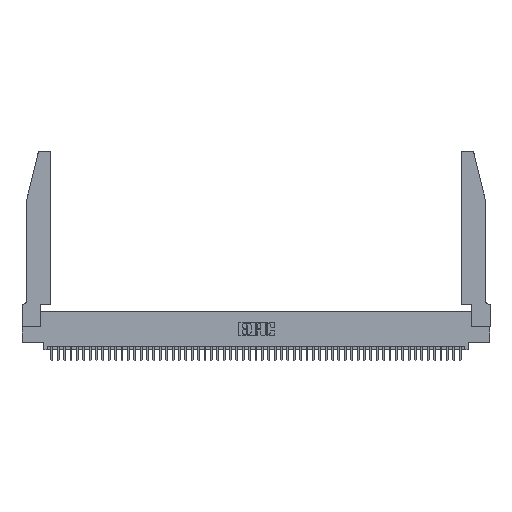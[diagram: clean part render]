
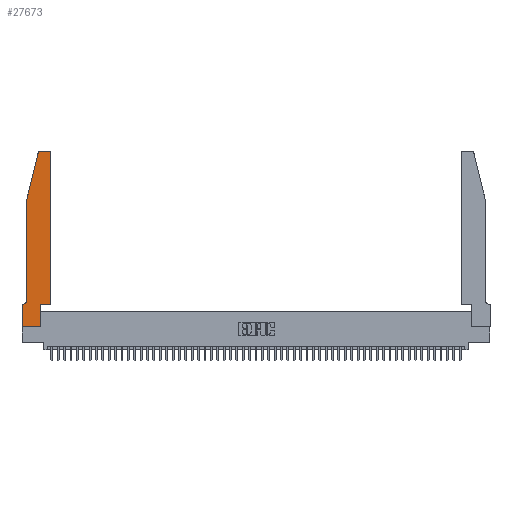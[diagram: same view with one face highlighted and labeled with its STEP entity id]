
A CAD part, top view. The second image highlights one B-rep face of the part: STEP entity #27673.
In plain terms, the highlighted planar face has unit normal (0, 0, 1).
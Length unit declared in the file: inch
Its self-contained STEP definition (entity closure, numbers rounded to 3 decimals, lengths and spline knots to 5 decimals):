
#548 = EDGE_CURVE ( 'NONE', #37580, #27733, #16621, .T. ) ;
#1304 = EDGE_CURVE ( 'NONE', #19321, #5507, #36340, .T. ) ;
#1772 = AXIS2_PLACEMENT_3D ( 'NONE', #45764, #21331, #49885 ) ;
#3377 = EDGE_CURVE ( 'NONE', #11514, #19321, #48997, .T. ) ;
#3870 = EDGE_CURVE ( 'NONE', #5507, #52704, #7978, .T. ) ;
#3989 = ORIENTED_EDGE ( 'NONE', *, *, #1304, .T. ) ;
#4039 = PLANE ( 'NONE',  #30158 ) ;
#5288 = EDGE_CURVE ( 'NONE', #27767, #37580, #44974, .T. ) ;
#5365 = EDGE_CURVE ( 'NONE', #30764, #27767, #31536, .T. ) ;
#5507 = VERTEX_POINT ( 'NONE', #20300 ) ;
#6475 = DIRECTION ( 'NONE',  ( 0., -1., 0. ) ) ;
#6552 = CARTESIAN_POINT ( 'NONE',  ( 0.4205, 2.75, 0.37 ) ) ;
#6656 = EDGE_CURVE ( 'NONE', #52704, #35107, #7088, .T. ) ;
#6718 = VERTEX_POINT ( 'NONE', #19467 ) ;
#7007 = CARTESIAN_POINT ( 'NONE',  ( 0., 0., 0.37 ) ) ;
#7088 = LINE ( 'NONE', #47504, #27619 ) ;
#7978 = CIRCLE ( 'NONE', #17635, 0.03 ) ;
#8817 = LINE ( 'NONE', #20969, #19744 ) ;
#9287 = ORIENTED_EDGE ( 'NONE', *, *, #5288, .T. ) ;
#9328 = ORIENTED_EDGE ( 'NONE', *, *, #3870, .T. ) ;
#9460 = CIRCLE ( 'NONE', #1772, 0.07 ) ;
#9462 = DIRECTION ( 'NONE',  ( 0., 0., 1. ) ) ;
#10316 = ORIENTED_EDGE ( 'NONE', *, *, #6656, .T. ) ;
#10530 = EDGE_CURVE ( 'NONE', #27733, #11514, #35978, .T. ) ;
#11138 = DIRECTION ( 'NONE',  ( 1., 0., 0. ) ) ;
#11514 = VERTEX_POINT ( 'NONE', #12403 ) ;
#11922 = CARTESIAN_POINT ( 'NONE',  ( 0.0755, 2., 0.37 ) ) ;
#12154 = ORIENTED_EDGE ( 'NONE', *, *, #10530, .T. ) ;
#12274 = CARTESIAN_POINT ( 'NONE',  ( 0., 0.35, 0.37 ) ) ;
#12403 = CARTESIAN_POINT ( 'NONE',  ( 0.4505, 2.72, 0.37 ) ) ;
#12608 = ORIENTED_EDGE ( 'NONE', *, *, #48501, .T. ) ;
#12703 = DIRECTION ( 'NONE',  ( -1., 0., 0. ) ) ;
#12795 = CARTESIAN_POINT ( 'NONE',  ( 0.4505, 0.35, 0.37 ) ) ;
#13423 = ORIENTED_EDGE ( 'NONE', *, *, #548, .T. ) ;
#13447 = ORIENTED_EDGE ( 'NONE', *, *, #5365, .T. ) ;
#14265 = VECTOR ( 'NONE', #16942, 39.37008 ) ;
#14744 = DIRECTION ( 'NONE',  ( 0., 0., 1. ) ) ;
#15454 = VERTEX_POINT ( 'NONE', #48443 ) ;
#16170 = CARTESIAN_POINT ( 'NONE',  ( 0.0755, 2., 0.37 ) ) ;
#16423 = DIRECTION ( 'NONE',  ( 1., 0., 0. ) ) ;
#16621 = LINE ( 'NONE', #50655, #37054 ) ;
#16942 = DIRECTION ( 'NONE',  ( 0., 1., 0. ) ) ;
#17635 = AXIS2_PLACEMENT_3D ( 'NONE', #33998, #9462, #38089 ) ;
#18958 = CARTESIAN_POINT ( 'NONE',  ( 0., 0., 0.37 ) ) ;
#18977 = EDGE_CURVE ( 'NONE', #6718, #42644, #8817, .T. ) ;
#19074 = DIRECTION ( 'NONE',  ( 0., 1., 0. ) ) ;
#19321 = VERTEX_POINT ( 'NONE', #6552 ) ;
#19467 = CARTESIAN_POINT ( 'NONE',  ( 0.0055, 0.35, 0.37 ) ) ;
#19744 = VECTOR ( 'NONE', #12703, 39.37008 ) ;
#19857 = LINE ( 'NONE', #16170, #39004 ) ;
#20300 = CARTESIAN_POINT ( 'NONE',  ( 0.284, 2.75, 0.37 ) ) ;
#20580 = CARTESIAN_POINT ( 'NONE',  ( 0.25487, 2.72718, 0.37 ) ) ;
#20799 = FACE_OUTER_BOUND ( 'NONE', #48003, .T. ) ;
#20892 = CARTESIAN_POINT ( 'NONE',  ( 0.2865, 0., 0.37 ) ) ;
#20969 = CARTESIAN_POINT ( 'NONE',  ( 0.0755, 0.35, 0.37 ) ) ;
#21331 = DIRECTION ( 'NONE',  ( 0., 0., -1. ) ) ;
#23020 = CARTESIAN_POINT ( 'NONE',  ( 0.2865, 0.35, 0.37 ) ) ;
#23251 = VECTOR ( 'NONE', #19074, 39.37008 ) ;
#24206 = VECTOR ( 'NONE', #26511, 39.37008 ) ;
#24578 = EDGE_CURVE ( 'NONE', #35107, #15454, #19857, .T. ) ;
#26511 = DIRECTION ( 'NONE',  ( -1., 0., 0. ) ) ;
#26944 = CARTESIAN_POINT ( 'NONE',  ( 0., 0., 0.37 ) ) ;
#27619 = VECTOR ( 'NONE', #43426, 39.37008 ) ;
#27673 = ADVANCED_FACE ( 'NONE', ( #20799 ), #4039, .T. ) ;
#27733 = VERTEX_POINT ( 'NONE', #41225 ) ;
#27767 = VERTEX_POINT ( 'NONE', #20892 ) ;
#28101 = EDGE_CURVE ( 'NONE', #42644, #30764, #41975, .T. ) ;
#30158 = AXIS2_PLACEMENT_3D ( 'NONE', #12274, #40871, #16423 ) ;
#30764 = VERTEX_POINT ( 'NONE', #18958 ) ;
#31098 = VECTOR ( 'NONE', #6475, 39.37008 ) ;
#31536 = LINE ( 'NONE', #7007, #51976 ) ;
#33998 = CARTESIAN_POINT ( 'NONE',  ( 0.284, 2.72, 0.37 ) ) ;
#34607 = CARTESIAN_POINT ( 'NONE',  ( 0., 0.35, 0.37 ) ) ;
#34696 = CARTESIAN_POINT ( 'NONE',  ( 0.2605, 2.75, 0.37 ) ) ;
#35107 = VERTEX_POINT ( 'NONE', #11922 ) ;
#35978 = LINE ( 'NONE', #12795, #14265 ) ;
#36061 = AXIS2_PLACEMENT_3D ( 'NONE', #39190, #14744, #43337 ) ;
#36340 = LINE ( 'NONE', #34696, #24206 ) ;
#37054 = VECTOR ( 'NONE', #46540, 39.37008 ) ;
#37580 = VERTEX_POINT ( 'NONE', #47078 ) ;
#38089 = DIRECTION ( 'NONE',  ( 1., 0., 0. ) ) ;
#39004 = VECTOR ( 'NONE', #48824, 39.37008 ) ;
#39190 = CARTESIAN_POINT ( 'NONE',  ( 0.4205, 2.72, 0.37 ) ) ;
#40871 = DIRECTION ( 'NONE',  ( 0., 0., 1. ) ) ;
#41225 = CARTESIAN_POINT ( 'NONE',  ( 0.4505, 0.35, 0.37 ) ) ;
#41975 = LINE ( 'NONE', #26944, #31098 ) ;
#42644 = VERTEX_POINT ( 'NONE', #34607 ) ;
#43337 = DIRECTION ( 'NONE',  ( 1., 0., 0. ) ) ;
#43342 = ORIENTED_EDGE ( 'NONE', *, *, #28101, .T. ) ;
#43426 = DIRECTION ( 'NONE',  ( -0.239, -0.971, 0. ) ) ;
#44151 = ORIENTED_EDGE ( 'NONE', *, *, #18977, .T. ) ;
#44974 = LINE ( 'NONE', #23020, #23251 ) ;
#45764 = CARTESIAN_POINT ( 'NONE',  ( 0.0055, 0.42, 0.37 ) ) ;
#46540 = DIRECTION ( 'NONE',  ( 1., 0., 0. ) ) ;
#47078 = CARTESIAN_POINT ( 'NONE',  ( 0.2865, 0.35, 0.37 ) ) ;
#47504 = CARTESIAN_POINT ( 'NONE',  ( 0.0755, 2., 0.37 ) ) ;
#48003 = EDGE_LOOP ( 'NONE', ( #3989, #9328, #10316, #51126, #12608, #44151, #43342, #13447, #9287, #13423, #12154, #48802 ) ) ;
#48443 = CARTESIAN_POINT ( 'NONE',  ( 0.0755, 0.42, 0.37 ) ) ;
#48501 = EDGE_CURVE ( 'NONE', #15454, #6718, #9460, .T. ) ;
#48802 = ORIENTED_EDGE ( 'NONE', *, *, #3377, .T. ) ;
#48824 = DIRECTION ( 'NONE',  ( 0., -1., 0. ) ) ;
#48997 = CIRCLE ( 'NONE', #36061, 0.03 ) ;
#49885 = DIRECTION ( 'NONE',  ( -1., 0., 0. ) ) ;
#50655 = CARTESIAN_POINT ( 'NONE',  ( 0.4505, 0.35, 0.37 ) ) ;
#51126 = ORIENTED_EDGE ( 'NONE', *, *, #24578, .T. ) ;
#51976 = VECTOR ( 'NONE', #11138, 39.37008 ) ;
#52704 = VERTEX_POINT ( 'NONE', #20580 ) ;
